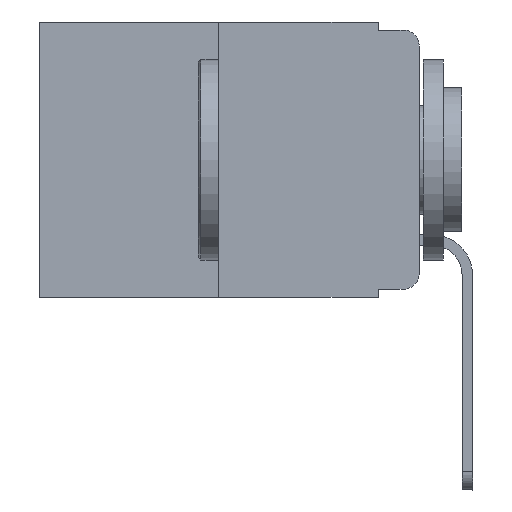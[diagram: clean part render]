
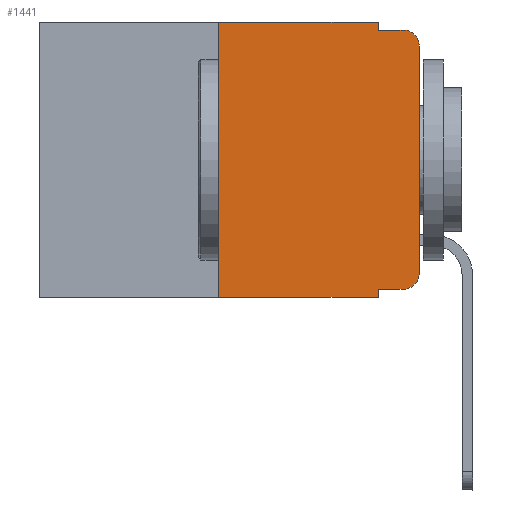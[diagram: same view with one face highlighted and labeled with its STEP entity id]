
A CAD part, left-side view. The second image highlights one B-rep face of the part: STEP entity #1441.
In plain terms, the highlighted planar face has unit normal (-1, 0, 0).
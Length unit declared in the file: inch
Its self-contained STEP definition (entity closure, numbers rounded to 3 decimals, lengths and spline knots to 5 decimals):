
#487 = EDGE_LOOP ( 'NONE', ( #6540, #6013, #7700, #2958, #5725, #8448, #5633, #695, #9770, #9662 ) ) ;
#695 = ORIENTED_EDGE ( 'NONE', *, *, #4463, .F. ) ;
#837 = VECTOR ( 'NONE', #6704, 39.37008 ) ;
#892 = CARTESIAN_POINT ( 'NONE',  ( 0., 0.02, -0.313 ) ) ;
#1110 = CARTESIAN_POINT ( 'NONE',  ( 0., 0.051, -0.343 ) ) ;
#1208 = VERTEX_POINT ( 'NONE', #3486 ) ;
#1255 = VECTOR ( 'NONE', #3030, 39.37008 ) ;
#1362 = VERTEX_POINT ( 'NONE', #7846 ) ;
#1441 = ADVANCED_FACE ( 'NONE', ( #4681 ), #8181, .F. ) ;
#1505 = EDGE_CURVE ( 'NONE', #3890, #3623, #10361, .T. ) ;
#1563 = CARTESIAN_POINT ( 'NONE',  ( 0., 0.02, -0.03 ) ) ;
#1688 = EDGE_CURVE ( 'NONE', #1362, #5584, #8386, .T. ) ;
#2107 = VERTEX_POINT ( 'NONE', #4311 ) ;
#2154 = CARTESIAN_POINT ( 'NONE',  ( 0., 0.25, 0. ) ) ;
#2341 = CIRCLE ( 'NONE', #6508, 0.02 ) ;
#2361 = VECTOR ( 'NONE', #7093, 39.37008 ) ;
#2556 = VECTOR ( 'NONE', #7633, 39.37008 ) ;
#2568 = CARTESIAN_POINT ( 'NONE',  ( 0., 0.051, 0. ) ) ;
#2710 = VERTEX_POINT ( 'NONE', #3368 ) ;
#2717 = CARTESIAN_POINT ( 'NONE',  ( 0., 0., -0.313 ) ) ;
#2958 = ORIENTED_EDGE ( 'NONE', *, *, #4302, .F. ) ;
#3004 = DIRECTION ( 'NONE',  ( 0., 0., -1. ) ) ;
#3030 = DIRECTION ( 'NONE',  ( 0., -1., 0. ) ) ;
#3267 = CARTESIAN_POINT ( 'NONE',  ( 0., 0.473, 0. ) ) ;
#3301 = VERTEX_POINT ( 'NONE', #2717 ) ;
#3368 = CARTESIAN_POINT ( 'NONE',  ( 0., 0.051, -0.01 ) ) ;
#3486 = CARTESIAN_POINT ( 'NONE',  ( 0., 0.051, 0. ) ) ;
#3623 = VERTEX_POINT ( 'NONE', #4257 ) ;
#3810 = LINE ( 'NONE', #2154, #6794 ) ;
#3860 = LINE ( 'NONE', #9589, #8217 ) ;
#3890 = VERTEX_POINT ( 'NONE', #10312 ) ;
#3912 = DIRECTION ( 'NONE',  ( 1., 0., 0. ) ) ;
#4048 = VERTEX_POINT ( 'NONE', #8962 ) ;
#4077 = CARTESIAN_POINT ( 'NONE',  ( 0., 0.051, -0.333 ) ) ;
#4257 = CARTESIAN_POINT ( 'NONE',  ( 0., 0.02, -0.01 ) ) ;
#4302 = EDGE_CURVE ( 'NONE', #1208, #2710, #8882, .T. ) ;
#4311 = CARTESIAN_POINT ( 'NONE',  ( 0., 0.25, -0.343 ) ) ;
#4463 = EDGE_CURVE ( 'NONE', #1362, #4549, #6645, .T. ) ;
#4549 = VERTEX_POINT ( 'NONE', #1110 ) ;
#4678 = EDGE_CURVE ( 'NONE', #2710, #3623, #9740, .T. ) ;
#4681 = FACE_OUTER_BOUND ( 'NONE', #487, .T. ) ;
#4736 = DIRECTION ( 'NONE',  ( 0., 0., 1. ) ) ;
#4936 = DIRECTION ( 'NONE',  ( -1., 0., 0. ) ) ;
#5305 = AXIS2_PLACEMENT_3D ( 'NONE', #7204, #3912, #9761 ) ;
#5379 = DIRECTION ( 'NONE',  ( 0., 0., -1. ) ) ;
#5440 = DIRECTION ( 'NONE',  ( 0., 0., 1. ) ) ;
#5584 = VERTEX_POINT ( 'NONE', #7210 ) ;
#5633 = ORIENTED_EDGE ( 'NONE', *, *, #8017, .T. ) ;
#5662 = DIRECTION ( 'NONE',  ( -1., 0., 0. ) ) ;
#5725 = ORIENTED_EDGE ( 'NONE', *, *, #8188, .F. ) ;
#6013 = ORIENTED_EDGE ( 'NONE', *, *, #1505, .T. ) ;
#6437 = CARTESIAN_POINT ( 'NONE',  ( 0., 0.051, 0. ) ) ;
#6441 = CARTESIAN_POINT ( 'NONE',  ( 0., 0.473, -0.343 ) ) ;
#6442 = VECTOR ( 'NONE', #5379, 39.37008 ) ;
#6508 = AXIS2_PLACEMENT_3D ( 'NONE', #892, #4936, #7352 ) ;
#6540 = ORIENTED_EDGE ( 'NONE', *, *, #6852, .T. ) ;
#6645 = LINE ( 'NONE', #2568, #9917 ) ;
#6704 = DIRECTION ( 'NONE',  ( 0., -1., 0. ) ) ;
#6794 = VECTOR ( 'NONE', #5440, 39.37008 ) ;
#6852 = EDGE_CURVE ( 'NONE', #3301, #3890, #3860, .T. ) ;
#7093 = DIRECTION ( 'NONE',  ( 0., -1., 0. ) ) ;
#7181 = CARTESIAN_POINT ( 'NONE',  ( 0., 0.051, -0.01 ) ) ;
#7204 = CARTESIAN_POINT ( 'NONE',  ( 0., 0.473, 0. ) ) ;
#7210 = CARTESIAN_POINT ( 'NONE',  ( 0., 0.02, -0.333 ) ) ;
#7352 = DIRECTION ( 'NONE',  ( 0., 0., -1. ) ) ;
#7633 = DIRECTION ( 'NONE',  ( 0., -1., 0. ) ) ;
#7700 = ORIENTED_EDGE ( 'NONE', *, *, #4678, .F. ) ;
#7846 = CARTESIAN_POINT ( 'NONE',  ( 0., 0.051, -0.333 ) ) ;
#8017 = EDGE_CURVE ( 'NONE', #2107, #4549, #10512, .T. ) ;
#8181 = PLANE ( 'NONE',  #5305 ) ;
#8188 = EDGE_CURVE ( 'NONE', #4048, #1208, #10737, .T. ) ;
#8217 = VECTOR ( 'NONE', #4736, 39.37008 ) ;
#8378 = DIRECTION ( 'NONE',  ( 0., 0., -1. ) ) ;
#8386 = LINE ( 'NONE', #4077, #2556 ) ;
#8448 = ORIENTED_EDGE ( 'NONE', *, *, #9309, .F. ) ;
#8553 = EDGE_CURVE ( 'NONE', #5584, #3301, #2341, .T. ) ;
#8882 = LINE ( 'NONE', #6437, #6442 ) ;
#8962 = CARTESIAN_POINT ( 'NONE',  ( 0., 0.25, 0. ) ) ;
#9309 = EDGE_CURVE ( 'NONE', #2107, #4048, #3810, .T. ) ;
#9589 = CARTESIAN_POINT ( 'NONE',  ( 0., 0., 0. ) ) ;
#9662 = ORIENTED_EDGE ( 'NONE', *, *, #8553, .T. ) ;
#9673 = AXIS2_PLACEMENT_3D ( 'NONE', #1563, #5662, #3004 ) ;
#9740 = LINE ( 'NONE', #7181, #1255 ) ;
#9761 = DIRECTION ( 'NONE',  ( 0., 0., -1. ) ) ;
#9770 = ORIENTED_EDGE ( 'NONE', *, *, #1688, .T. ) ;
#9917 = VECTOR ( 'NONE', #8378, 39.37008 ) ;
#10312 = CARTESIAN_POINT ( 'NONE',  ( 0., 0., -0.03 ) ) ;
#10361 = CIRCLE ( 'NONE', #9673, 0.02 ) ;
#10512 = LINE ( 'NONE', #6441, #2361 ) ;
#10737 = LINE ( 'NONE', #3267, #837 ) ;
